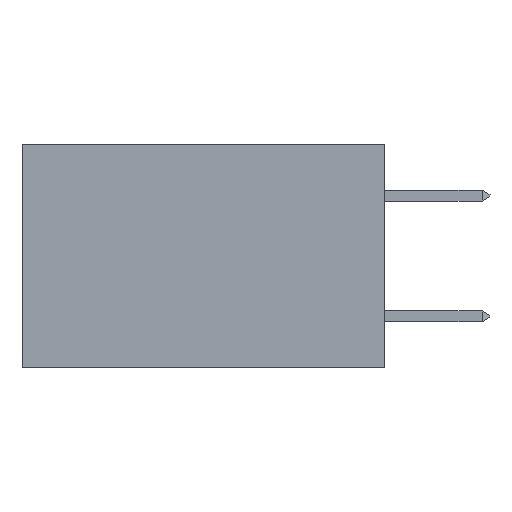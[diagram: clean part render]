
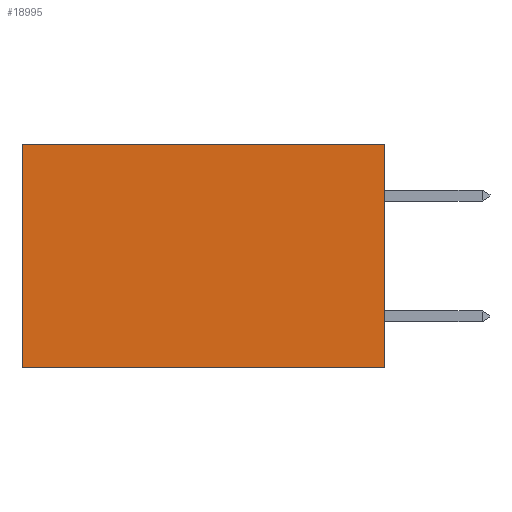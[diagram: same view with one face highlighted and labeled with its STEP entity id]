
A CAD part, left-side view. The second image highlights one B-rep face of the part: STEP entity #18995.
In plain terms, the highlighted planar face has unit normal (-1, 0, 0).
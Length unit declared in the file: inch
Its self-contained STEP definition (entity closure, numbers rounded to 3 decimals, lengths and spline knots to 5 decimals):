
#141 = AXIS2_PLACEMENT_3D ( 'NONE', #13895, #14134, #4629 ) ;
#1178 = CARTESIAN_POINT ( 'NONE',  ( 0.2875, 0.6, -0.37 ) ) ;
#2827 = DIRECTION ( 'NONE',  ( 0., 1., 0. ) ) ;
#3039 = VERTEX_POINT ( 'NONE', #1178 ) ;
#4481 = ORIENTED_EDGE ( 'NONE', *, *, #16340, .T. ) ;
#4629 = DIRECTION ( 'NONE',  ( 0., 0., -1. ) ) ;
#4823 = DIRECTION ( 'NONE',  ( 0., 0., -1. ) ) ;
#5576 = VECTOR ( 'NONE', #4823, 39.37008 ) ;
#5731 = CARTESIAN_POINT ( 'NONE',  ( 0.2875, 0., -0.37 ) ) ;
#6020 = CARTESIAN_POINT ( 'NONE',  ( 0.2875, 0.6, 0. ) ) ;
#6217 = ORIENTED_EDGE ( 'NONE', *, *, #10795, .T. ) ;
#6364 = VECTOR ( 'NONE', #22504, 39.37008 ) ;
#7331 = EDGE_LOOP ( 'NONE', ( #4481, #15724, #11847, #6217 ) ) ;
#7611 = DIRECTION ( 'NONE',  ( 0., 1., 0. ) ) ;
#8094 = EDGE_CURVE ( 'NONE', #10735, #3039, #17777, .T. ) ;
#8684 = FACE_OUTER_BOUND ( 'NONE', #7331, .T. ) ;
#10143 = CARTESIAN_POINT ( 'NONE',  ( 0.2875, 0., 0. ) ) ;
#10735 = VERTEX_POINT ( 'NONE', #5731 ) ;
#10795 = EDGE_CURVE ( 'NONE', #20066, #14067, #13713, .T. ) ;
#11847 = ORIENTED_EDGE ( 'NONE', *, *, #23597, .F. ) ;
#13391 = LINE ( 'NONE', #14924, #6364 ) ;
#13713 = LINE ( 'NONE', #14822, #15471 ) ;
#13895 = CARTESIAN_POINT ( 'NONE',  ( 0.2875, 0., 0. ) ) ;
#14067 = VERTEX_POINT ( 'NONE', #6020 ) ;
#14134 = DIRECTION ( 'NONE',  ( 1., 0., 0. ) ) ;
#14822 = CARTESIAN_POINT ( 'NONE',  ( 0.2875, 0., 0. ) ) ;
#14924 = CARTESIAN_POINT ( 'NONE',  ( 0.2875, 0., 0. ) ) ;
#15471 = VECTOR ( 'NONE', #7611, 39.37008 ) ;
#15724 = ORIENTED_EDGE ( 'NONE', *, *, #8094, .F. ) ;
#15960 = CARTESIAN_POINT ( 'NONE',  ( 0.2875, 0., -0.37 ) ) ;
#16340 = EDGE_CURVE ( 'NONE', #14067, #3039, #24067, .T. ) ;
#17777 = LINE ( 'NONE', #15960, #18959 ) ;
#18959 = VECTOR ( 'NONE', #2827, 39.37008 ) ;
#18995 = ADVANCED_FACE ( 'NONE', ( #8684 ), #23599, .F. ) ;
#20066 = VERTEX_POINT ( 'NONE', #10143 ) ;
#21578 = CARTESIAN_POINT ( 'NONE',  ( 0.2875, 0.6, 0. ) ) ;
#22504 = DIRECTION ( 'NONE',  ( 0., 0., -1. ) ) ;
#23597 = EDGE_CURVE ( 'NONE', #20066, #10735, #13391, .T. ) ;
#23599 = PLANE ( 'NONE',  #141 ) ;
#24067 = LINE ( 'NONE', #21578, #5576 ) ;
